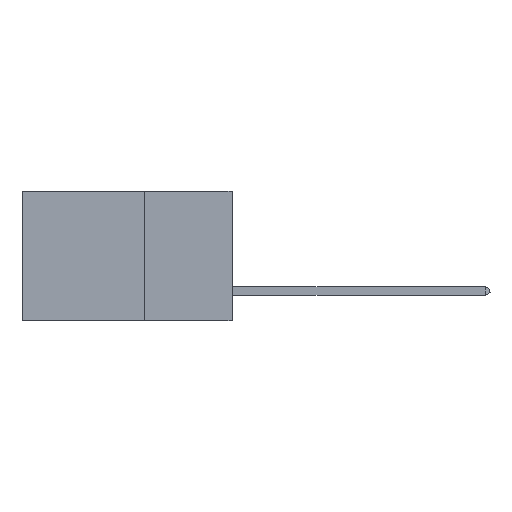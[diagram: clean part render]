
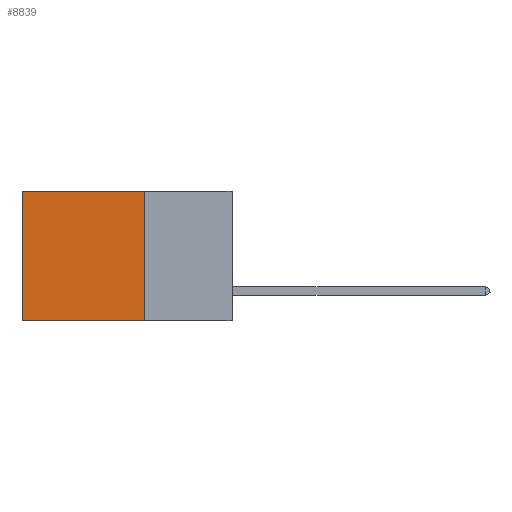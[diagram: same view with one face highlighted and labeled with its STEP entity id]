
A CAD part, left-side view. The second image highlights one B-rep face of the part: STEP entity #8839.
In plain terms, the highlighted planar face has unit normal (-1, 0, 0).
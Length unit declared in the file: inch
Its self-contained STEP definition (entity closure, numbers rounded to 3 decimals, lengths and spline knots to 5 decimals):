
#1374 = LINE ( 'NONE', #28585, #13205 ) ;
#3542 = EDGE_CURVE ( 'NONE', #6508, #31691, #25054, .T. ) ;
#4624 = CARTESIAN_POINT ( 'NONE',  ( 0.2875, 0.6, 0. ) ) ;
#6495 = LINE ( 'NONE', #29648, #27864 ) ;
#6508 = VERTEX_POINT ( 'NONE', #16124 ) ;
#7891 = DIRECTION ( 'NONE',  ( 1., 0., 0. ) ) ;
#8595 = DIRECTION ( 'NONE',  ( 0., 0., -1. ) ) ;
#8839 = ADVANCED_FACE ( 'NONE', ( #12719 ), #21438, .F. ) ;
#10803 = DIRECTION ( 'NONE',  ( 0., 0., -1. ) ) ;
#12491 = ORIENTED_EDGE ( 'NONE', *, *, #15233, .F. ) ;
#12696 = ORIENTED_EDGE ( 'NONE', *, *, #28391, .F. ) ;
#12719 = FACE_OUTER_BOUND ( 'NONE', #34049, .T. ) ;
#13205 = VECTOR ( 'NONE', #31880, 39.37008 ) ;
#15233 = EDGE_CURVE ( 'NONE', #6508, #26557, #6495, .T. ) ;
#15351 = EDGE_CURVE ( 'NONE', #31691, #29287, #26145, .T. ) ;
#15898 = CARTESIAN_POINT ( 'NONE',  ( 0.2875, 0.25, -0.37 ) ) ;
#16124 = CARTESIAN_POINT ( 'NONE',  ( 0.2875, 0.25, 0. ) ) ;
#18690 = DIRECTION ( 'NONE',  ( 0., 0., -1. ) ) ;
#18830 = CARTESIAN_POINT ( 'NONE',  ( 0.2875, 0.25, 0. ) ) ;
#18945 = DIRECTION ( 'NONE',  ( 0., 1., 0. ) ) ;
#19017 = VECTOR ( 'NONE', #18945, 39.37008 ) ;
#21438 = PLANE ( 'NONE',  #25557 ) ;
#24161 = CARTESIAN_POINT ( 'NONE',  ( 0.2875, 0.6, -0.37 ) ) ;
#24203 = CARTESIAN_POINT ( 'NONE',  ( 0.2875, 0.25, 0. ) ) ;
#24478 = CARTESIAN_POINT ( 'NONE',  ( 0.2875, 0.6, 0. ) ) ;
#25054 = LINE ( 'NONE', #18830, #19017 ) ;
#25557 = AXIS2_PLACEMENT_3D ( 'NONE', #24203, #7891, #8595 ) ;
#26145 = LINE ( 'NONE', #24478, #27408 ) ;
#26557 = VERTEX_POINT ( 'NONE', #15898 ) ;
#26648 = ORIENTED_EDGE ( 'NONE', *, *, #3542, .T. ) ;
#27408 = VECTOR ( 'NONE', #10803, 39.37008 ) ;
#27864 = VECTOR ( 'NONE', #18690, 39.37008 ) ;
#28391 = EDGE_CURVE ( 'NONE', #26557, #29287, #1374, .T. ) ;
#28585 = CARTESIAN_POINT ( 'NONE',  ( 0.2875, 0.25, -0.37 ) ) ;
#29287 = VERTEX_POINT ( 'NONE', #24161 ) ;
#29648 = CARTESIAN_POINT ( 'NONE',  ( 0.2875, 0.25, 0. ) ) ;
#31691 = VERTEX_POINT ( 'NONE', #4624 ) ;
#31880 = DIRECTION ( 'NONE',  ( 0., 1., 0. ) ) ;
#33530 = ORIENTED_EDGE ( 'NONE', *, *, #15351, .T. ) ;
#34049 = EDGE_LOOP ( 'NONE', ( #33530, #12696, #12491, #26648 ) ) ;
